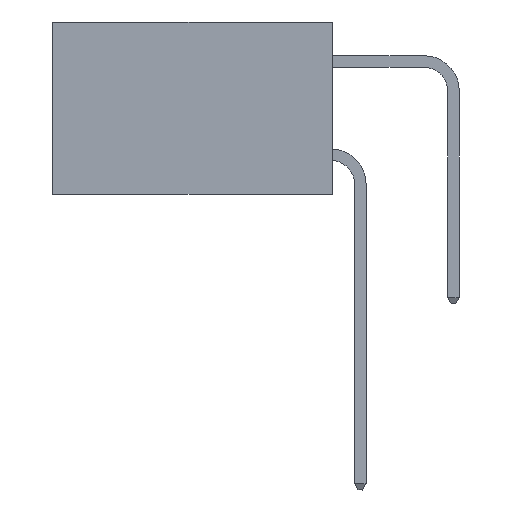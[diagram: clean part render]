
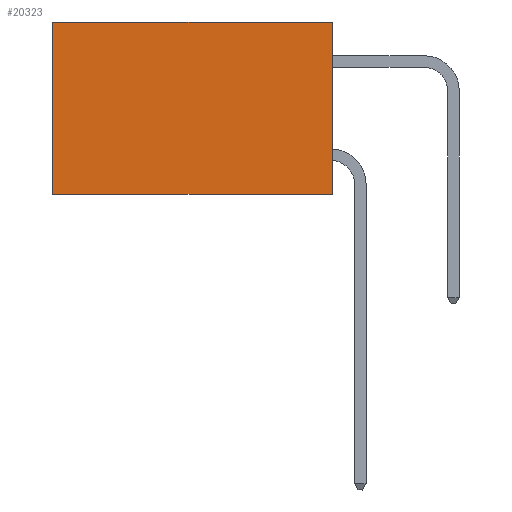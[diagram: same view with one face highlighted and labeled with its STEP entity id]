
A CAD part, left-side view. The second image highlights one B-rep face of the part: STEP entity #20323.
In plain terms, the highlighted planar face has unit normal (-1, 0, 0).
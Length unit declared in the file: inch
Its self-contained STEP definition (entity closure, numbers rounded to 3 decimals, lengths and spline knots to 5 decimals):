
#1606 = LINE ( 'NONE', #6302, #24090 ) ;
#2765 = LINE ( 'NONE', #25590, #27737 ) ;
#3729 = DIRECTION ( 'NONE',  ( 0., 1., 0. ) ) ;
#4397 = ORIENTED_EDGE ( 'NONE', *, *, #23891, .T. ) ;
#5828 = EDGE_CURVE ( 'NONE', #8337, #16474, #1606, .T. ) ;
#6302 = CARTESIAN_POINT ( 'NONE',  ( 0.298, 0., -0.37 ) ) ;
#6410 = EDGE_LOOP ( 'NONE', ( #4397, #11279, #12724, #13866 ) ) ;
#7473 = CARTESIAN_POINT ( 'NONE',  ( 0.298, 0.6, 0. ) ) ;
#8295 = AXIS2_PLACEMENT_3D ( 'NONE', #22682, #27323, #9632 ) ;
#8337 = VERTEX_POINT ( 'NONE', #15876 ) ;
#9346 = LINE ( 'NONE', #14910, #12408 ) ;
#9632 = DIRECTION ( 'NONE',  ( 0., 0., -1. ) ) ;
#10181 = CARTESIAN_POINT ( 'NONE',  ( 0.298, 0.6, 0. ) ) ;
#10288 = CARTESIAN_POINT ( 'NONE',  ( 0.298, 0., 0. ) ) ;
#10765 = EDGE_CURVE ( 'NONE', #14029, #15529, #2765, .T. ) ;
#11279 = ORIENTED_EDGE ( 'NONE', *, *, #5828, .F. ) ;
#12408 = VECTOR ( 'NONE', #23788, 39.37008 ) ;
#12592 = VECTOR ( 'NONE', #12658, 39.37008 ) ;
#12658 = DIRECTION ( 'NONE',  ( 0., 0., -1. ) ) ;
#12724 = ORIENTED_EDGE ( 'NONE', *, *, #27517, .F. ) ;
#13866 = ORIENTED_EDGE ( 'NONE', *, *, #10765, .T. ) ;
#14029 = VERTEX_POINT ( 'NONE', #10288 ) ;
#14910 = CARTESIAN_POINT ( 'NONE',  ( 0.298, 0., 0. ) ) ;
#15529 = VERTEX_POINT ( 'NONE', #7473 ) ;
#15876 = CARTESIAN_POINT ( 'NONE',  ( 0.298, 0., -0.37 ) ) ;
#16474 = VERTEX_POINT ( 'NONE', #27818 ) ;
#20071 = LINE ( 'NONE', #10181, #12592 ) ;
#20323 = ADVANCED_FACE ( 'NONE', ( #21265 ), #20478, .F. ) ;
#20478 = PLANE ( 'NONE',  #8295 ) ;
#21265 = FACE_OUTER_BOUND ( 'NONE', #6410, .T. ) ;
#22682 = CARTESIAN_POINT ( 'NONE',  ( 0.298, 0., 0. ) ) ;
#23265 = DIRECTION ( 'NONE',  ( 0., 1., 0. ) ) ;
#23788 = DIRECTION ( 'NONE',  ( 0., 0., -1. ) ) ;
#23891 = EDGE_CURVE ( 'NONE', #15529, #16474, #20071, .T. ) ;
#24090 = VECTOR ( 'NONE', #23265, 39.37008 ) ;
#25590 = CARTESIAN_POINT ( 'NONE',  ( 0.298, 0., 0. ) ) ;
#27323 = DIRECTION ( 'NONE',  ( 1., 0., 0. ) ) ;
#27517 = EDGE_CURVE ( 'NONE', #14029, #8337, #9346, .T. ) ;
#27737 = VECTOR ( 'NONE', #3729, 39.37008 ) ;
#27818 = CARTESIAN_POINT ( 'NONE',  ( 0.298, 0.6, -0.37 ) ) ;
